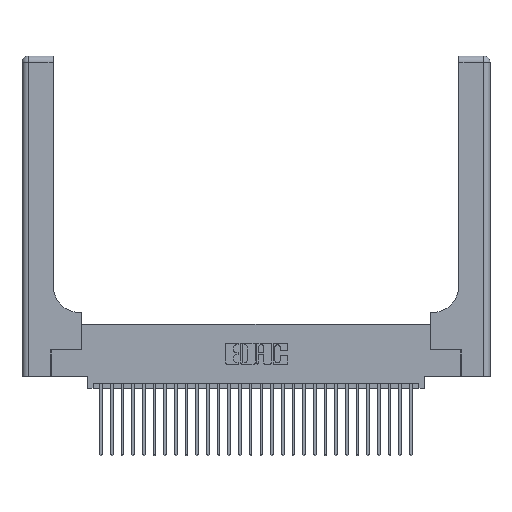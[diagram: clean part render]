
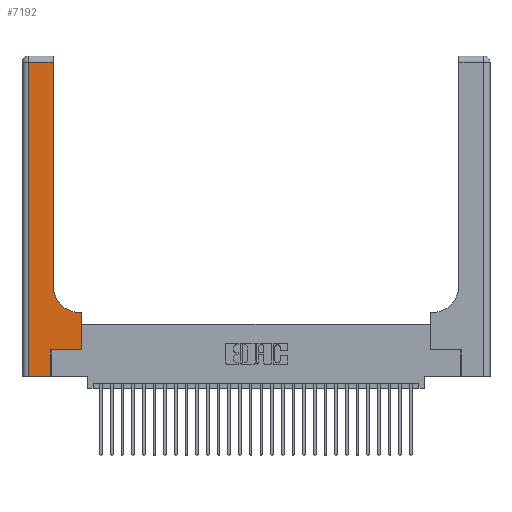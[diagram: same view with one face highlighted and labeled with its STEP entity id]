
A CAD part, top view. The second image highlights one B-rep face of the part: STEP entity #7192.
In plain terms, the highlighted planar face has unit normal (0, 0, 1).
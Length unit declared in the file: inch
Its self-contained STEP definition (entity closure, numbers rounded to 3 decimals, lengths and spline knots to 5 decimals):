
#247 = CARTESIAN_POINT ( 'NONE',  ( 0.2915, 0.85, 0.37 ) ) ;
#300 = VERTEX_POINT ( 'NONE', #22737 ) ;
#380 = VERTEX_POINT ( 'NONE', #8938 ) ;
#485 = DIRECTION ( 'NONE',  ( 0., 1., 0. ) ) ;
#761 = EDGE_CURVE ( 'NONE', #18760, #11321, #28573, .T. ) ;
#1041 = DIRECTION ( 'NONE',  ( -1., 0., 0. ) ) ;
#1381 = VECTOR ( 'NONE', #17133, 39.37008 ) ;
#4242 = VECTOR ( 'NONE', #28184, 39.37008 ) ;
#4297 = EDGE_CURVE ( 'NONE', #26768, #9076, #14247, .T. ) ;
#4336 = VERTEX_POINT ( 'NONE', #25003 ) ;
#4788 = EDGE_CURVE ( 'NONE', #9076, #4336, #5731, .T. ) ;
#4870 = DIRECTION ( 'NONE',  ( 0., -1., 0. ) ) ;
#5052 = ORIENTED_EDGE ( 'NONE', *, *, #12360, .T. ) ;
#5202 = VECTOR ( 'NONE', #1041, 39.37008 ) ;
#5731 = LINE ( 'NONE', #7728, #9423 ) ;
#5867 = DIRECTION ( 'NONE',  ( 0., 0., -1. ) ) ;
#6263 = AXIS2_PLACEMENT_3D ( 'NONE', #15405, #5867, #17404 ) ;
#6343 = VECTOR ( 'NONE', #4870, 39.37008 ) ;
#6976 = CARTESIAN_POINT ( 'NONE',  ( 0.5585, 0.25, 0.37 ) ) ;
#7192 = ADVANCED_FACE ( 'NONE', ( #20726 ), #24973, .F. ) ;
#7429 = CARTESIAN_POINT ( 'NONE',  ( 0.269, 0.25, 0.37 ) ) ;
#7649 = EDGE_CURVE ( 'NONE', #15229, #380, #26574, .T. ) ;
#7728 = CARTESIAN_POINT ( 'NONE',  ( 0.2915, 3., 0.37 ) ) ;
#7961 = EDGE_CURVE ( 'NONE', #11321, #26768, #28802, .T. ) ;
#8799 = DIRECTION ( 'NONE',  ( 0., 1., 0. ) ) ;
#8938 = CARTESIAN_POINT ( 'NONE',  ( 0.06, 0., 0.37 ) ) ;
#9076 = VERTEX_POINT ( 'NONE', #247 ) ;
#9280 = CARTESIAN_POINT ( 'NONE',  ( 0.5585, 0.6, 0.37 ) ) ;
#9423 = VECTOR ( 'NONE', #485, 39.37008 ) ;
#9749 = LINE ( 'NONE', #25467, #25558 ) ;
#10806 = VERTEX_POINT ( 'NONE', #7429 ) ;
#11321 = VERTEX_POINT ( 'NONE', #9280 ) ;
#11545 = VECTOR ( 'NONE', #13267, 39.37008 ) ;
#11843 = ORIENTED_EDGE ( 'NONE', *, *, #4297, .T. ) ;
#12360 = EDGE_CURVE ( 'NONE', #10806, #18760, #24461, .T. ) ;
#12678 = DIRECTION ( 'NONE',  ( 1., 0., 0. ) ) ;
#13267 = DIRECTION ( 'NONE',  ( 1., 0., 0. ) ) ;
#13470 = CARTESIAN_POINT ( 'NONE',  ( 0.06, 3., 0.37 ) ) ;
#13526 = ORIENTED_EDGE ( 'NONE', *, *, #7649, .T. ) ;
#14247 = CIRCLE ( 'NONE', #6263, 0.25 ) ;
#15229 = VERTEX_POINT ( 'NONE', #28283 ) ;
#15365 = LINE ( 'NONE', #26552, #27113 ) ;
#15405 = CARTESIAN_POINT ( 'NONE',  ( 0.5415, 0.85, 0.37 ) ) ;
#15625 = ORIENTED_EDGE ( 'NONE', *, *, #24454, .T. ) ;
#16120 = ORIENTED_EDGE ( 'NONE', *, *, #26514, .T. ) ;
#17133 = DIRECTION ( 'NONE',  ( -1., 0., 0. ) ) ;
#17404 = DIRECTION ( 'NONE',  ( 1., 0., 0. ) ) ;
#17526 = EDGE_CURVE ( 'NONE', #380, #300, #15365, .T. ) ;
#18537 = AXIS2_PLACEMENT_3D ( 'NONE', #22897, #20920, #27718 ) ;
#18760 = VERTEX_POINT ( 'NONE', #25445 ) ;
#19871 = CARTESIAN_POINT ( 'NONE',  ( 0.5415, 0.6, 0.37 ) ) ;
#20065 = ORIENTED_EDGE ( 'NONE', *, *, #761, .T. ) ;
#20160 = CARTESIAN_POINT ( 'NONE',  ( 0.269, 0.25, 0.37 ) ) ;
#20726 = FACE_OUTER_BOUND ( 'NONE', #23191, .T. ) ;
#20794 = ORIENTED_EDGE ( 'NONE', *, *, #4788, .T. ) ;
#20920 = DIRECTION ( 'NONE',  ( 0., 0., -1. ) ) ;
#21593 = ORIENTED_EDGE ( 'NONE', *, *, #7961, .T. ) ;
#22737 = CARTESIAN_POINT ( 'NONE',  ( 0.269, 0., 0.37 ) ) ;
#22897 = CARTESIAN_POINT ( 'NONE',  ( 0., 3., 0.37 ) ) ;
#23191 = EDGE_LOOP ( 'NONE', ( #20794, #15625, #13526, #24195, #16120, #5052, #20065, #21593, #11843 ) ) ;
#24035 = CARTESIAN_POINT ( 'NONE',  ( 0., 2.94, 0.37 ) ) ;
#24195 = ORIENTED_EDGE ( 'NONE', *, *, #17526, .T. ) ;
#24454 = EDGE_CURVE ( 'NONE', #4336, #15229, #26050, .T. ) ;
#24461 = LINE ( 'NONE', #20160, #11545 ) ;
#24973 = PLANE ( 'NONE',  #18537 ) ;
#25003 = CARTESIAN_POINT ( 'NONE',  ( 0.2915, 2.94, 0.37 ) ) ;
#25445 = CARTESIAN_POINT ( 'NONE',  ( 0.5585, 0.25, 0.37 ) ) ;
#25467 = CARTESIAN_POINT ( 'NONE',  ( 0.269, 0., 0.37 ) ) ;
#25558 = VECTOR ( 'NONE', #8799, 39.37008 ) ;
#26050 = LINE ( 'NONE', #24035, #1381 ) ;
#26514 = EDGE_CURVE ( 'NONE', #300, #10806, #9749, .T. ) ;
#26552 = CARTESIAN_POINT ( 'NONE',  ( 0., 0., 0.37 ) ) ;
#26574 = LINE ( 'NONE', #13470, #6343 ) ;
#26768 = VERTEX_POINT ( 'NONE', #19871 ) ;
#27113 = VECTOR ( 'NONE', #12678, 39.37008 ) ;
#27214 = CARTESIAN_POINT ( 'NONE',  ( 0.2915, 0.6, 0.37 ) ) ;
#27718 = DIRECTION ( 'NONE',  ( -1., 0., 0. ) ) ;
#28184 = DIRECTION ( 'NONE',  ( 0., 1., 0. ) ) ;
#28283 = CARTESIAN_POINT ( 'NONE',  ( 0.06, 2.94, 0.37 ) ) ;
#28573 = LINE ( 'NONE', #6976, #4242 ) ;
#28802 = LINE ( 'NONE', #27214, #5202 ) ;
